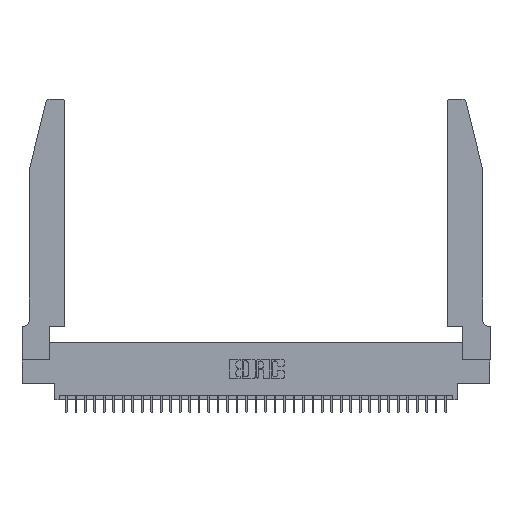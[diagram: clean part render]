
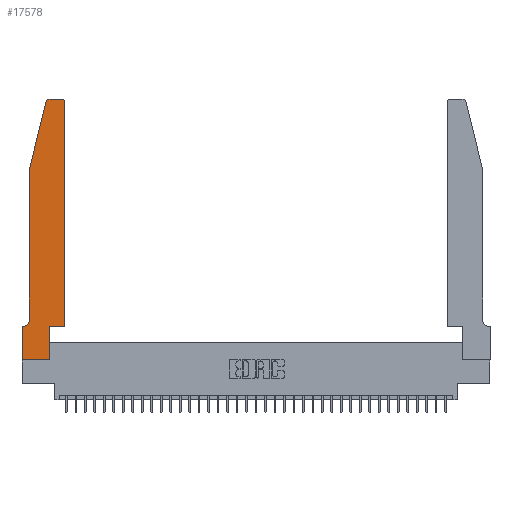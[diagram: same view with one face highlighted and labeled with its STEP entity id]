
A CAD part, top view. The second image highlights one B-rep face of the part: STEP entity #17578.
In plain terms, the highlighted planar face has unit normal (0, 0, 1).
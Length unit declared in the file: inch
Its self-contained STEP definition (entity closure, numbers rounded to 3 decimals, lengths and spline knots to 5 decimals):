
#89 = CARTESIAN_POINT ( 'NONE',  ( 0.0055, 0.42, 0.37 ) ) ;
#532 = CARTESIAN_POINT ( 'NONE',  ( 0.0755, 2., 0.37 ) ) ;
#733 = DIRECTION ( 'NONE',  ( 0., -1., 0. ) ) ;
#787 = CARTESIAN_POINT ( 'NONE',  ( 0.4505, 0.35, 0.37 ) ) ;
#792 = EDGE_CURVE ( 'NONE', #35150, #27847, #29622, .T. ) ;
#801 = VERTEX_POINT ( 'NONE', #17587 ) ;
#921 = CARTESIAN_POINT ( 'NONE',  ( 0.0755, 2., 0.37 ) ) ;
#1491 = CARTESIAN_POINT ( 'NONE',  ( 0.0755, 0.35, 0.37 ) ) ;
#1987 = CARTESIAN_POINT ( 'NONE',  ( 0., 0.35, 0.37 ) ) ;
#2184 = EDGE_CURVE ( 'NONE', #801, #17410, #23802, .T. ) ;
#2216 = CARTESIAN_POINT ( 'NONE',  ( 0.0755, 0.42, 0.37 ) ) ;
#2629 = EDGE_CURVE ( 'NONE', #28165, #35150, #23389, .T. ) ;
#2883 = EDGE_CURVE ( 'NONE', #13625, #5071, #25427, .T. ) ;
#3613 = EDGE_CURVE ( 'NONE', #20703, #28165, #5113, .T. ) ;
#3975 = CARTESIAN_POINT ( 'NONE',  ( 0.2865, 0., 0.37 ) ) ;
#4046 = ORIENTED_EDGE ( 'NONE', *, *, #26865, .T. ) ;
#4583 = CARTESIAN_POINT ( 'NONE',  ( 0.284, 2.72, 0.37 ) ) ;
#5015 = PLANE ( 'NONE',  #33818 ) ;
#5071 = VERTEX_POINT ( 'NONE', #33774 ) ;
#5113 = CIRCLE ( 'NONE', #28626, 0.03 ) ;
#5856 = VECTOR ( 'NONE', #21332, 39.37008 ) ;
#6104 = ORIENTED_EDGE ( 'NONE', *, *, #12980, .T. ) ;
#6756 = VECTOR ( 'NONE', #20442, 39.37008 ) ;
#7010 = ORIENTED_EDGE ( 'NONE', *, *, #7555, .T. ) ;
#7071 = VECTOR ( 'NONE', #7871, 39.37008 ) ;
#7292 = FACE_OUTER_BOUND ( 'NONE', #31619, .T. ) ;
#7479 = DIRECTION ( 'NONE',  ( 1., 0., 0. ) ) ;
#7523 = EDGE_CURVE ( 'NONE', #5071, #21225, #23281, .T. ) ;
#7555 = EDGE_CURVE ( 'NONE', #21225, #33014, #26655, .T. ) ;
#7871 = DIRECTION ( 'NONE',  ( 0., 1., 0. ) ) ;
#8020 = DIRECTION ( 'NONE',  ( 0., 0., -1. ) ) ;
#8545 = DIRECTION ( 'NONE',  ( -1., 0., 0. ) ) ;
#8654 = LINE ( 'NONE', #8833, #13143 ) ;
#8829 = VERTEX_POINT ( 'NONE', #22909 ) ;
#8833 = CARTESIAN_POINT ( 'NONE',  ( 0., 0., 0.37 ) ) ;
#9058 = LINE ( 'NONE', #15096, #28832 ) ;
#9634 = EDGE_CURVE ( 'NONE', #8829, #20703, #33831, .T. ) ;
#10339 = ORIENTED_EDGE ( 'NONE', *, *, #24842, .T. ) ;
#11009 = DIRECTION ( 'NONE',  ( 0., 0., 1. ) ) ;
#11894 = AXIS2_PLACEMENT_3D ( 'NONE', #89, #8020, #19543 ) ;
#12225 = ORIENTED_EDGE ( 'NONE', *, *, #7523, .T. ) ;
#12596 = EDGE_CURVE ( 'NONE', #17410, #14573, #9058, .T. ) ;
#12683 = ORIENTED_EDGE ( 'NONE', *, *, #2184, .T. ) ;
#12775 = DIRECTION ( 'NONE',  ( 0., 0., 1. ) ) ;
#12980 = EDGE_CURVE ( 'NONE', #14573, #13625, #8654, .T. ) ;
#13143 = VECTOR ( 'NONE', #28262, 39.37008 ) ;
#13625 = VERTEX_POINT ( 'NONE', #3975 ) ;
#14337 = VECTOR ( 'NONE', #34892, 39.37008 ) ;
#14573 = VERTEX_POINT ( 'NONE', #27474 ) ;
#15096 = CARTESIAN_POINT ( 'NONE',  ( 0., 0., 0.37 ) ) ;
#15184 = ORIENTED_EDGE ( 'NONE', *, *, #792, .T. ) ;
#16812 = VECTOR ( 'NONE', #8545, 39.37008 ) ;
#17410 = VERTEX_POINT ( 'NONE', #32047 ) ;
#17578 = ADVANCED_FACE ( 'NONE', ( #7292 ), #5015, .T. ) ;
#17587 = CARTESIAN_POINT ( 'NONE',  ( 0.0055, 0.35, 0.37 ) ) ;
#18029 = CIRCLE ( 'NONE', #23443, 0.03 ) ;
#18448 = CARTESIAN_POINT ( 'NONE',  ( 0.25487, 2.72718, 0.37 ) ) ;
#19326 = DIRECTION ( 'NONE',  ( 0., 0., 1. ) ) ;
#19474 = ORIENTED_EDGE ( 'NONE', *, *, #3613, .T. ) ;
#19543 = DIRECTION ( 'NONE',  ( -1., 0., 0. ) ) ;
#20442 = DIRECTION ( 'NONE',  ( 0., 1., 0. ) ) ;
#20703 = VERTEX_POINT ( 'NONE', #25036 ) ;
#21225 = VERTEX_POINT ( 'NONE', #31686 ) ;
#21332 = DIRECTION ( 'NONE',  ( -1., 0., 0. ) ) ;
#22766 = ORIENTED_EDGE ( 'NONE', *, *, #9634, .T. ) ;
#22909 = CARTESIAN_POINT ( 'NONE',  ( 0.4205, 2.75, 0.37 ) ) ;
#23103 = DIRECTION ( 'NONE',  ( 1., 0., 0. ) ) ;
#23281 = LINE ( 'NONE', #26469, #24244 ) ;
#23389 = LINE ( 'NONE', #532, #14337 ) ;
#23443 = AXIS2_PLACEMENT_3D ( 'NONE', #25355, #11009, #23103 ) ;
#23802 = LINE ( 'NONE', #1491, #5856 ) ;
#24244 = VECTOR ( 'NONE', #34778, 39.37008 ) ;
#24842 = EDGE_CURVE ( 'NONE', #27847, #801, #28785, .T. ) ;
#25036 = CARTESIAN_POINT ( 'NONE',  ( 0.284, 2.75, 0.37 ) ) ;
#25355 = CARTESIAN_POINT ( 'NONE',  ( 0.4205, 2.72, 0.37 ) ) ;
#25427 = LINE ( 'NONE', #33727, #7071 ) ;
#26397 = ORIENTED_EDGE ( 'NONE', *, *, #12596, .T. ) ;
#26469 = CARTESIAN_POINT ( 'NONE',  ( 0.4505, 0.35, 0.37 ) ) ;
#26655 = LINE ( 'NONE', #787, #6756 ) ;
#26865 = EDGE_CURVE ( 'NONE', #33014, #8829, #18029, .T. ) ;
#27474 = CARTESIAN_POINT ( 'NONE',  ( 0., 0., 0.37 ) ) ;
#27847 = VERTEX_POINT ( 'NONE', #2216 ) ;
#27883 = CARTESIAN_POINT ( 'NONE',  ( 0.0755, 2., 0.37 ) ) ;
#28165 = VERTEX_POINT ( 'NONE', #18448 ) ;
#28262 = DIRECTION ( 'NONE',  ( 1., 0., 0. ) ) ;
#28626 = AXIS2_PLACEMENT_3D ( 'NONE', #4583, #19326, #35912 ) ;
#28785 = CIRCLE ( 'NONE', #11894, 0.07 ) ;
#28832 = VECTOR ( 'NONE', #733, 39.37008 ) ;
#29323 = ORIENTED_EDGE ( 'NONE', *, *, #2883, .T. ) ;
#29622 = LINE ( 'NONE', #921, #32316 ) ;
#31619 = EDGE_LOOP ( 'NONE', ( #22766, #19474, #34679, #15184, #10339, #12683, #26397, #6104, #29323, #12225, #7010, #4046 ) ) ;
#31686 = CARTESIAN_POINT ( 'NONE',  ( 0.4505, 0.35, 0.37 ) ) ;
#32047 = CARTESIAN_POINT ( 'NONE',  ( 0., 0.35, 0.37 ) ) ;
#32086 = DIRECTION ( 'NONE',  ( 0., -1., 0. ) ) ;
#32316 = VECTOR ( 'NONE', #32086, 39.37008 ) ;
#33014 = VERTEX_POINT ( 'NONE', #33693 ) ;
#33693 = CARTESIAN_POINT ( 'NONE',  ( 0.4505, 2.72, 0.37 ) ) ;
#33727 = CARTESIAN_POINT ( 'NONE',  ( 0.2865, 0.35, 0.37 ) ) ;
#33774 = CARTESIAN_POINT ( 'NONE',  ( 0.2865, 0.35, 0.37 ) ) ;
#33818 = AXIS2_PLACEMENT_3D ( 'NONE', #1987, #12775, #7479 ) ;
#33831 = LINE ( 'NONE', #37036, #16812 ) ;
#34679 = ORIENTED_EDGE ( 'NONE', *, *, #2629, .T. ) ;
#34778 = DIRECTION ( 'NONE',  ( 1., 0., 0. ) ) ;
#34892 = DIRECTION ( 'NONE',  ( -0.239, -0.971, 0. ) ) ;
#35150 = VERTEX_POINT ( 'NONE', #27883 ) ;
#35912 = DIRECTION ( 'NONE',  ( 1., 0., 0. ) ) ;
#37036 = CARTESIAN_POINT ( 'NONE',  ( 0.2605, 2.75, 0.37 ) ) ;
